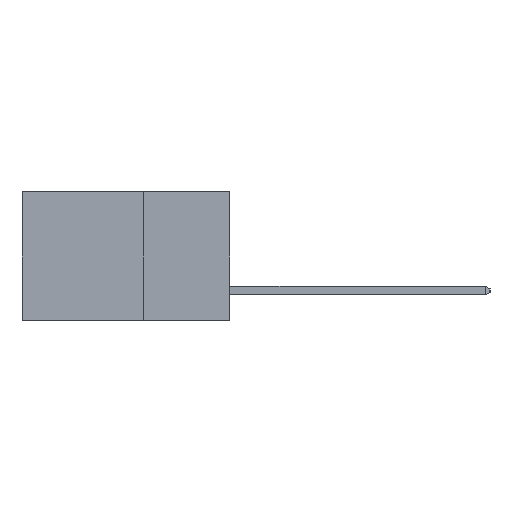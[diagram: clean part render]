
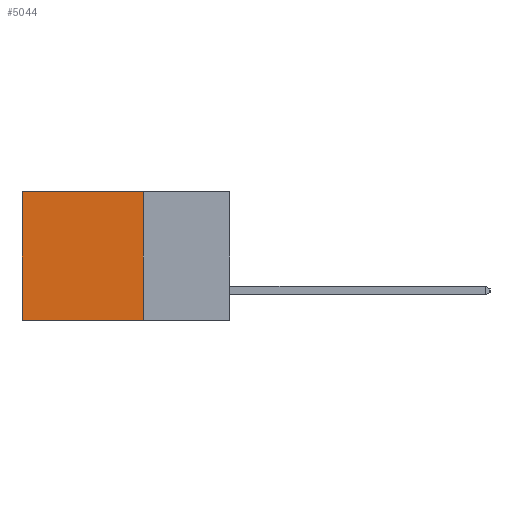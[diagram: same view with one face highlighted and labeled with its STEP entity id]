
A CAD part, left-side view. The second image highlights one B-rep face of the part: STEP entity #5044.
In plain terms, the highlighted planar face has unit normal (-1, 0, 0).
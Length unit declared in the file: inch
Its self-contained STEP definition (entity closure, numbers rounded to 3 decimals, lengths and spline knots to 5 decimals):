
#402 = CARTESIAN_POINT ( 'NONE',  ( 0.2615, 0.25, -0.37 ) ) ;
#557 = EDGE_CURVE ( 'NONE', #12741, #2985, #22402, .T. ) ;
#2431 = DIRECTION ( 'NONE',  ( 0., 1., 0. ) ) ;
#2515 = LINE ( 'NONE', #23131, #12655 ) ;
#2761 = CARTESIAN_POINT ( 'NONE',  ( 0.2615, 0.6, -0.37 ) ) ;
#2785 = DIRECTION ( 'NONE',  ( 0., 0., -1. ) ) ;
#2948 = CARTESIAN_POINT ( 'NONE',  ( 0.2615, 0.25, -0.37 ) ) ;
#2985 = VERTEX_POINT ( 'NONE', #15296 ) ;
#3673 = EDGE_LOOP ( 'NONE', ( #16367, #24065, #7165, #6713 ) ) ;
#5044 = ADVANCED_FACE ( 'NONE', ( #8527 ), #10697, .F. ) ;
#5396 = VERTEX_POINT ( 'NONE', #2948 ) ;
#6713 = ORIENTED_EDGE ( 'NONE', *, *, #24640, .T. ) ;
#6746 = CARTESIAN_POINT ( 'NONE',  ( 0.2615, 0.25, 0. ) ) ;
#7165 = ORIENTED_EDGE ( 'NONE', *, *, #15523, .F. ) ;
#8102 = VERTEX_POINT ( 'NONE', #24809 ) ;
#8527 = FACE_OUTER_BOUND ( 'NONE', #3673, .T. ) ;
#8789 = DIRECTION ( 'NONE',  ( 0., 1., 0. ) ) ;
#9228 = DIRECTION ( 'NONE',  ( 0., 0., -1. ) ) ;
#10301 = DIRECTION ( 'NONE',  ( 0., 0., -1. ) ) ;
#10355 = DIRECTION ( 'NONE',  ( 1., 0., 0. ) ) ;
#10586 = CARTESIAN_POINT ( 'NONE',  ( 0.2615, 0.25, -0.37 ) ) ;
#10697 = PLANE ( 'NONE',  #25688 ) ;
#12655 = VECTOR ( 'NONE', #9228, 39.37008 ) ;
#12741 = VERTEX_POINT ( 'NONE', #20452 ) ;
#15296 = CARTESIAN_POINT ( 'NONE',  ( 0.2615, 0.6, -0.37 ) ) ;
#15523 = EDGE_CURVE ( 'NONE', #8102, #5396, #2515, .T. ) ;
#16367 = ORIENTED_EDGE ( 'NONE', *, *, #557, .T. ) ;
#16570 = VECTOR ( 'NONE', #2785, 39.37008 ) ;
#17337 = VECTOR ( 'NONE', #2431, 39.37008 ) ;
#17481 = VECTOR ( 'NONE', #8789, 39.37008 ) ;
#20452 = CARTESIAN_POINT ( 'NONE',  ( 0.2615, 0.6, 0. ) ) ;
#20972 = EDGE_CURVE ( 'NONE', #5396, #2985, #21927, .T. ) ;
#21927 = LINE ( 'NONE', #402, #17337 ) ;
#22402 = LINE ( 'NONE', #2761, #16570 ) ;
#22699 = LINE ( 'NONE', #6746, #17481 ) ;
#23131 = CARTESIAN_POINT ( 'NONE',  ( 0.2615, 0.25, -0.37 ) ) ;
#24065 = ORIENTED_EDGE ( 'NONE', *, *, #20972, .F. ) ;
#24640 = EDGE_CURVE ( 'NONE', #8102, #12741, #22699, .T. ) ;
#24809 = CARTESIAN_POINT ( 'NONE',  ( 0.2615, 0.25, 0. ) ) ;
#25688 = AXIS2_PLACEMENT_3D ( 'NONE', #10586, #10355, #10301 ) ;
